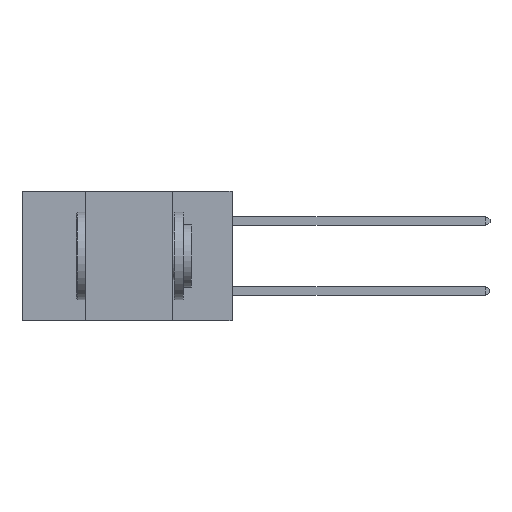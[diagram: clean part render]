
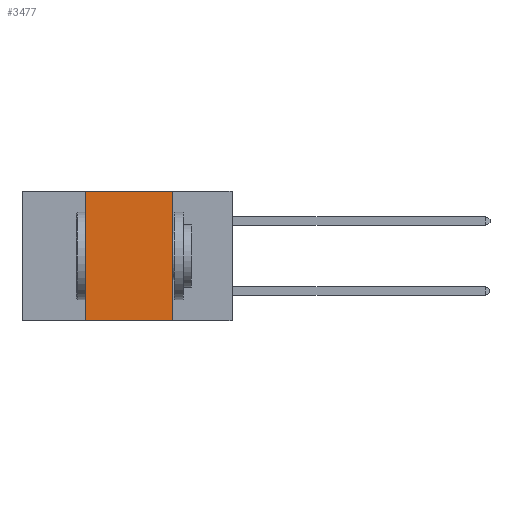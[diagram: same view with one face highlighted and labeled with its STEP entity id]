
A CAD part, left-side view. The second image highlights one B-rep face of the part: STEP entity #3477.
In plain terms, the highlighted planar face has unit normal (-1, 0, 0).
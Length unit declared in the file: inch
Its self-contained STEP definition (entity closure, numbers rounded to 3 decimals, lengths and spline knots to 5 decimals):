
#862 = EDGE_CURVE ( 'NONE', #8770, #1879, #7268, .T. ) ;
#1023 = EDGE_CURVE ( 'NONE', #9327, #1879, #5237, .T. ) ;
#1594 = ORIENTED_EDGE ( 'NONE', *, *, #862, .F. ) ;
#1879 = VERTEX_POINT ( 'NONE', #9503 ) ;
#2201 = VECTOR ( 'NONE', #7865, 39.37008 ) ;
#2495 = CARTESIAN_POINT ( 'NONE',  ( 0., 0.6, 0. ) ) ;
#3106 = ORIENTED_EDGE ( 'NONE', *, *, #1023, .T. ) ;
#3477 = ADVANCED_FACE ( 'NONE', ( #8021 ), #7665, .F. ) ;
#3616 = DIRECTION ( 'NONE',  ( 0., -1., 0. ) ) ;
#3835 = ORIENTED_EDGE ( 'NONE', *, *, #8462, .F. ) ;
#4220 = ORIENTED_EDGE ( 'NONE', *, *, #10726, .F. ) ;
#4724 = AXIS2_PLACEMENT_3D ( 'NONE', #7744, #8639, #7525 ) ;
#5237 = LINE ( 'NONE', #13209, #2201 ) ;
#5523 = CARTESIAN_POINT ( 'NONE',  ( 0., 0.42, 0. ) ) ;
#6167 = LINE ( 'NONE', #2495, #11238 ) ;
#7168 = VECTOR ( 'NONE', #11639, 39.37008 ) ;
#7217 = CARTESIAN_POINT ( 'NONE',  ( 0., 0.42, -0.37 ) ) ;
#7268 = LINE ( 'NONE', #13424, #9370 ) ;
#7525 = DIRECTION ( 'NONE',  ( 0., 0., -1. ) ) ;
#7665 = PLANE ( 'NONE',  #4724 ) ;
#7744 = CARTESIAN_POINT ( 'NONE',  ( 0., 0.6, 0. ) ) ;
#7865 = DIRECTION ( 'NONE',  ( 0., -1., 0. ) ) ;
#8021 = FACE_OUTER_BOUND ( 'NONE', #13513, .T. ) ;
#8462 = EDGE_CURVE ( 'NONE', #9327, #12120, #9895, .T. ) ;
#8639 = DIRECTION ( 'NONE',  ( 1., 0., 0. ) ) ;
#8770 = VERTEX_POINT ( 'NONE', #10687 ) ;
#9327 = VERTEX_POINT ( 'NONE', #7217 ) ;
#9370 = VECTOR ( 'NONE', #12404, 39.37008 ) ;
#9503 = CARTESIAN_POINT ( 'NONE',  ( 0., 0.17, -0.37 ) ) ;
#9895 = LINE ( 'NONE', #10658, #7168 ) ;
#10658 = CARTESIAN_POINT ( 'NONE',  ( 0., 0.42, 0. ) ) ;
#10687 = CARTESIAN_POINT ( 'NONE',  ( 0., 0.17, 0. ) ) ;
#10726 = EDGE_CURVE ( 'NONE', #12120, #8770, #6167, .T. ) ;
#11238 = VECTOR ( 'NONE', #3616, 39.37008 ) ;
#11639 = DIRECTION ( 'NONE',  ( 0., 0., 1. ) ) ;
#12120 = VERTEX_POINT ( 'NONE', #5523 ) ;
#12404 = DIRECTION ( 'NONE',  ( 0., 0., -1. ) ) ;
#13209 = CARTESIAN_POINT ( 'NONE',  ( 0., 0.6, -0.37 ) ) ;
#13424 = CARTESIAN_POINT ( 'NONE',  ( 0., 0.17, 0. ) ) ;
#13513 = EDGE_LOOP ( 'NONE', ( #1594, #4220, #3835, #3106 ) ) ;
